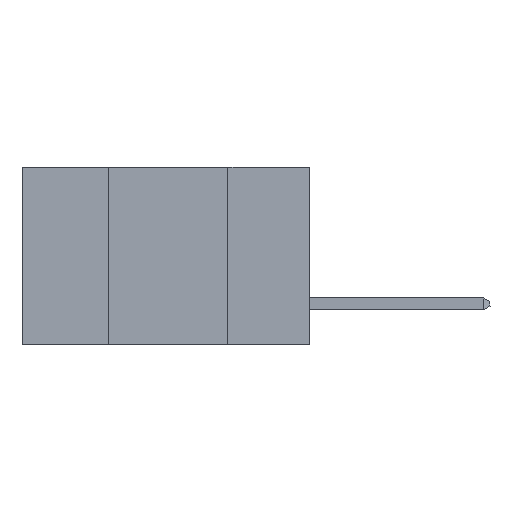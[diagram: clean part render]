
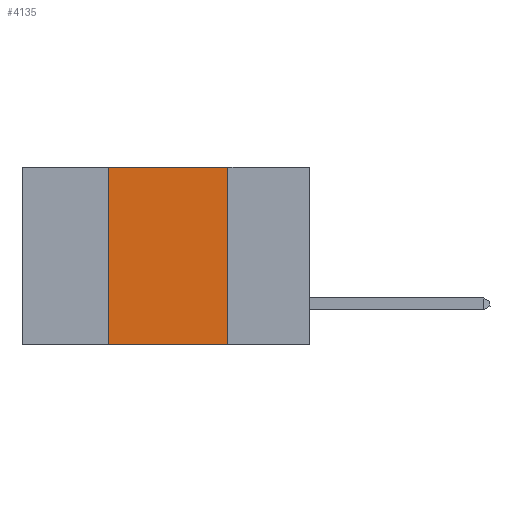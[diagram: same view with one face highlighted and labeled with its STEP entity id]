
A CAD part, left-side view. The second image highlights one B-rep face of the part: STEP entity #4135.
In plain terms, the highlighted planar face has unit normal (-1, 0, 0).
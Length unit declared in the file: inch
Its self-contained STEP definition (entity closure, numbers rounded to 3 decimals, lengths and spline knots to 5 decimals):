
#1410 = CARTESIAN_POINT ( 'NONE',  ( 0., 0.6, 0. ) ) ;
#1732 = CARTESIAN_POINT ( 'NONE',  ( 0., 0.42, 0. ) ) ;
#2572 = LINE ( 'NONE', #5379, #5640 ) ;
#3164 = DIRECTION ( 'NONE',  ( 0., -1., 0. ) ) ;
#3863 = CARTESIAN_POINT ( 'NONE',  ( 0., 0.17, -0.37 ) ) ;
#3865 = DIRECTION ( 'NONE',  ( 0., 0., -1. ) ) ;
#4135 = ADVANCED_FACE ( 'NONE', ( #12255 ), #5950, .F. ) ;
#4911 = AXIS2_PLACEMENT_3D ( 'NONE', #1410, #16427, #7479 ) ;
#5128 = VECTOR ( 'NONE', #17336, 39.37008 ) ;
#5379 = CARTESIAN_POINT ( 'NONE',  ( 0., 0.17, 0. ) ) ;
#5640 = VECTOR ( 'NONE', #3865, 39.37008 ) ;
#5678 = LINE ( 'NONE', #1732, #17129 ) ;
#5950 = PLANE ( 'NONE',  #4911 ) ;
#6215 = CARTESIAN_POINT ( 'NONE',  ( 0., 0.17, 0. ) ) ;
#6284 = EDGE_CURVE ( 'NONE', #13314, #17152, #9125, .T. ) ;
#7308 = EDGE_CURVE ( 'NONE', #14568, #17527, #7422, .T. ) ;
#7422 = LINE ( 'NONE', #12164, #16316 ) ;
#7479 = DIRECTION ( 'NONE',  ( 0., 0., -1. ) ) ;
#8071 = ORIENTED_EDGE ( 'NONE', *, *, #7308, .F. ) ;
#8104 = ORIENTED_EDGE ( 'NONE', *, *, #15443, .F. ) ;
#8412 = CARTESIAN_POINT ( 'NONE',  ( 0., 0.6, -0.37 ) ) ;
#9125 = LINE ( 'NONE', #8412, #5128 ) ;
#9157 = CARTESIAN_POINT ( 'NONE',  ( 0., 0.42, -0.37 ) ) ;
#10971 = EDGE_LOOP ( 'NONE', ( #8104, #8071, #17472, #16433 ) ) ;
#12164 = CARTESIAN_POINT ( 'NONE',  ( 0., 0.6, 0. ) ) ;
#12255 = FACE_OUTER_BOUND ( 'NONE', #10971, .T. ) ;
#13314 = VERTEX_POINT ( 'NONE', #9157 ) ;
#14568 = VERTEX_POINT ( 'NONE', #17978 ) ;
#15443 = EDGE_CURVE ( 'NONE', #17527, #17152, #2572, .T. ) ;
#16316 = VECTOR ( 'NONE', #3164, 39.37008 ) ;
#16427 = DIRECTION ( 'NONE',  ( 1., 0., 0. ) ) ;
#16433 = ORIENTED_EDGE ( 'NONE', *, *, #6284, .T. ) ;
#17129 = VECTOR ( 'NONE', #18236, 39.37008 ) ;
#17152 = VERTEX_POINT ( 'NONE', #3863 ) ;
#17336 = DIRECTION ( 'NONE',  ( 0., -1., 0. ) ) ;
#17472 = ORIENTED_EDGE ( 'NONE', *, *, #18060, .F. ) ;
#17527 = VERTEX_POINT ( 'NONE', #6215 ) ;
#17978 = CARTESIAN_POINT ( 'NONE',  ( 0., 0.42, 0. ) ) ;
#18060 = EDGE_CURVE ( 'NONE', #13314, #14568, #5678, .T. ) ;
#18236 = DIRECTION ( 'NONE',  ( 0., 0., 1. ) ) ;
